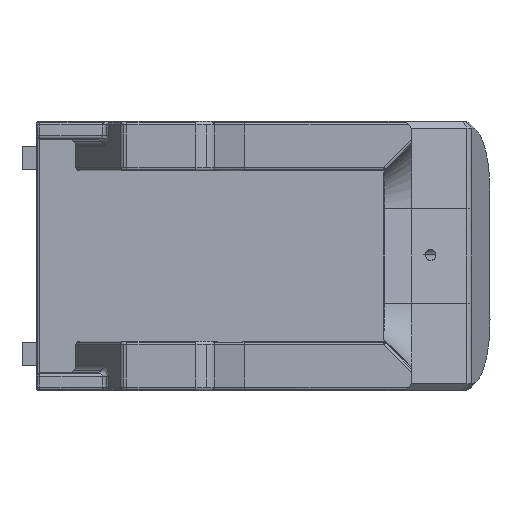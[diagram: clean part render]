
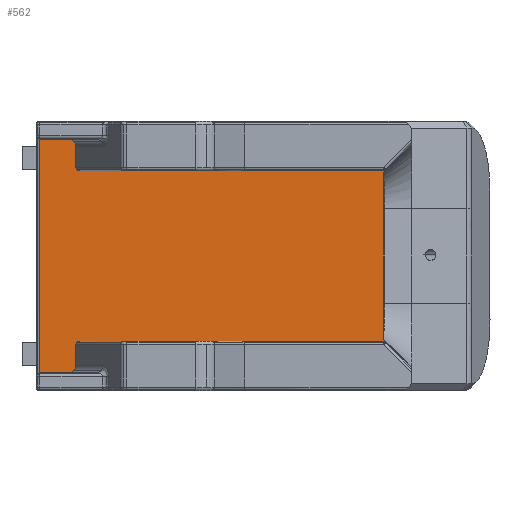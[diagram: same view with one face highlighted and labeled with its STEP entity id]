
A CAD part, left-side view. The second image highlights one B-rep face of the part: STEP entity #562.
In plain terms, the highlighted planar face has unit normal (-1, 0, 0).
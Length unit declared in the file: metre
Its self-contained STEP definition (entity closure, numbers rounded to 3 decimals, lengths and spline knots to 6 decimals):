
#562=ADVANCED_FACE('0:72',(#1731),#1732,.F.);
#1731=FACE_OUTER_BOUND('',#7564,.T.);
#1732=PLANE('',#7565);
#7564=EDGE_LOOP('',(#12483,#12484,#12485,#12486,#12487,#12488,#12489,#12490,#12491,#12492,#12493,#12494,#12495,#12496,#12497,#12498,#12499,#12500,#12501,#12502,#12503,#12504));
#7565=AXIS2_PLACEMENT_3D('',#12505,#12506,#12507);
#12483=ORIENTED_EDGE('',*,*,#14951,.F.);
#12484=ORIENTED_EDGE('',*,*,#13797,.F.);
#12485=ORIENTED_EDGE('',*,*,#14913,.F.);
#12486=ORIENTED_EDGE('',*,*,#14964,.T.);
#12487=ORIENTED_EDGE('',*,*,#14910,.T.);
#12488=ORIENTED_EDGE('',*,*,#13803,.T.);
#12489=ORIENTED_EDGE('',*,*,#15021,.F.);
#12490=ORIENTED_EDGE('',*,*,#15022,.F.);
#12491=ORIENTED_EDGE('',*,*,#15023,.F.);
#12492=ORIENTED_EDGE('',*,*,#13785,.T.);
#12493=ORIENTED_EDGE('',*,*,#14929,.T.);
#12494=ORIENTED_EDGE('',*,*,#15024,.T.);
#12495=ORIENTED_EDGE('',*,*,#14930,.F.);
#12496=ORIENTED_EDGE('',*,*,#13783,.F.);
#12497=ORIENTED_EDGE('',*,*,#15025,.F.);
#12498=ORIENTED_EDGE('',*,*,#13758,.F.);
#12499=ORIENTED_EDGE('',*,*,#14950,.F.);
#12500=ORIENTED_EDGE('',*,*,#15026,.F.);
#12501=ORIENTED_EDGE('',*,*,#14947,.T.);
#12502=ORIENTED_EDGE('',*,*,#14957,.F.);
#12503=ORIENTED_EDGE('',*,*,#13805,.F.);
#12504=ORIENTED_EDGE('',*,*,#14909,.F.);
#12505=CARTESIAN_POINT('',(-0.16753,-0.031141,0.001));
#12506=DIRECTION('',(1.0,0.,0.));
#12507=DIRECTION('',(0.,1.0,0.0));
#13758=EDGE_CURVE('0:1620',#15643,#15646,#15647,.T.);
#13783=EDGE_CURVE('0:1833',#15688,#15684,#15690,.T.);
#13785=EDGE_CURVE('0:1827',#15694,#15691,#15695,.T.);
#13797=EDGE_CURVE('0:1809',#15714,#15717,#15718,.T.);
#13803=EDGE_CURVE('0:1815',#15723,#15727,#15729,.T.);
#13805=EDGE_CURVE('0:1722',#15730,#15733,#15734,.T.);
#14909=EDGE_CURVE('0:1722',#17521,#15730,#17523,.T.);
#14910=EDGE_CURVE('0:1815',#17524,#15723,#17525,.T.);
#14913=EDGE_CURVE('0:1809',#17527,#15714,#17529,.T.);
#14929=EDGE_CURVE('0:1827',#15691,#17549,#17551,.T.);
#14930=EDGE_CURVE('0:1833',#15684,#17552,#17553,.T.);
#14947=EDGE_CURVE('0:1839',#17577,#17575,#17578,.T.);
#14950=EDGE_CURVE('0:1620',#17580,#15643,#17582,.T.);
#14951=EDGE_CURVE('0:1758',#15717,#17521,#17583,.T.);
#14957=EDGE_CURVE('0:1842',#15733,#17575,#17590,.T.);
#14964=EDGE_CURVE('0:1812',#17527,#17524,#17598,.T.);
#15021=EDGE_CURVE('0:1818',#15328,#15727,#17685,.T.);
#15022=EDGE_CURVE('0:1821',#17686,#15328,#17687,.T.);
#15023=EDGE_CURVE('0:1824',#15694,#17686,#17688,.T.);
#15024=EDGE_CURVE('0:1830',#17549,#17552,#17689,.T.);
#15025=EDGE_CURVE('0:1836',#15646,#15688,#17690,.T.);
#15026=EDGE_CURVE('0:1641',#17577,#17580,#17691,.T.);
#15328=VERTEX_POINT('NONE',#18089);
#15643=VERTEX_POINT('',#18612);
#15646=VERTEX_POINT('NONE',#18616);
#15647=CIRCLE('',#18617,0.0005);
#15684=VERTEX_POINT('',#18672);
#15688=VERTEX_POINT('NONE',#18677);
#15690=ELLIPSE('',#18680,0.000577,0.0005);
#15691=VERTEX_POINT('',#18681);
#15694=VERTEX_POINT('NONE',#18685);
#15695=ELLIPSE('',#18686,0.001155,0.001);
#15714=VERTEX_POINT('',#18725);
#15717=VERTEX_POINT('NONE',#18729);
#15718=ELLIPSE('',#18730,0.000577,0.0005);
#15723=VERTEX_POINT('',#18736);
#15727=VERTEX_POINT('NONE',#18745);
#15729=ELLIPSE('',#18748,0.001155,0.001);
#15730=VERTEX_POINT('',#18749);
#15733=VERTEX_POINT('NONE',#18753);
#15734=CIRCLE('',#18754,0.0005);
#17521=VERTEX_POINT('NONE',#23033);
#17523=CIRCLE('',#23036,0.0005);
#17524=VERTEX_POINT('NONE',#23037);
#17525=ELLIPSE('',#23038,0.001155,0.001);
#17527=VERTEX_POINT('NONE',#23041);
#17529=ELLIPSE('',#23044,0.000577,0.0005);
#17549=VERTEX_POINT('NONE',#23093);
#17551=ELLIPSE('',#23096,0.001155,0.001);
#17552=VERTEX_POINT('NONE',#23097);
#17553=ELLIPSE('',#23098,0.000577,0.0005);
#17575=VERTEX_POINT('NONE',#23129);
#17577=VERTEX_POINT('NONE',#23132);
#17578=LINE('',#23133,#23134);
#17580=VERTEX_POINT('NONE',#23137);
#17582=CIRCLE('',#23140,0.0005);
#17583=LINE('',#23141,#23142);
#17590=LINE('',#23155,#23156);
#17598=LINE('',#23168,#23169);
#17685=LINE('',#23385,#23386);
#17686=VERTEX_POINT('NONE',#23387);
#17687=LINE('',#23388,#23389);
#17688=LINE('',#23390,#23391);
#17689=LINE('',#23392,#23393);
#17690=LINE('',#23394,#23395);
#17691=LINE('',#23396,#23397);
#18089=CARTESIAN_POINT('',(-0.16753,-0.00879,0.0175));
#18612=CARTESIAN_POINT('',(-0.16753,-0.057524,-0.011038));
#18616=CARTESIAN_POINT('',(-0.16753,-0.057332,-0.011));
#18617=AXIS2_PLACEMENT_3D('',#24233,#24234,#24235);
#18672=CARTESIAN_POINT('',(-0.16753,-0.014076,-0.011146));
#18677=CARTESIAN_POINT('',(-0.16753,-0.014485,-0.011));
#18680=AXIS2_PLACEMENT_3D('',#24280,#24281,#24282);
#18681=CARTESIAN_POINT('',(-0.16753,-0.013569,-0.015207));
#18685=CARTESIAN_POINT('',(-0.16753,-0.012753,-0.0155));
#18686=AXIS2_PLACEMENT_3D('',#24284,#24285,#24286);
#18725=CARTESIAN_POINT('',(-0.16753,-0.014076,0.013146));
#18729=CARTESIAN_POINT('',(-0.16753,-0.014485,0.013));
#18730=AXIS2_PLACEMENT_3D('',#24299,#24300,#24301);
#18736=CARTESIAN_POINT('',(-0.16753,-0.013569,0.017207));
#18745=CARTESIAN_POINT('',(-0.16753,-0.012753,0.0175));
#18748=AXIS2_PLACEMENT_3D('',#24308,#24309,#24310);
#18749=CARTESIAN_POINT('',(-0.16753,-0.057524,0.013038));
#18753=CARTESIAN_POINT('',(-0.16753,-0.057686,0.013146));
#18754=AXIS2_PLACEMENT_3D('',#24312,#24313,#24314);
#23033=CARTESIAN_POINT('',(-0.16753,-0.057333,0.013));
#23036=AXIS2_PLACEMENT_3D('',#26068,#26069,#26070);
#23037=CARTESIAN_POINT('',(-0.16753,-0.013907,0.0165));
#23038=AXIS2_PLACEMENT_3D('',#26071,#26072,#26073);
#23041=CARTESIAN_POINT('',(-0.16753,-0.013907,0.0135));
#23044=AXIS2_PLACEMENT_3D('',#26076,#26077,#26078);
#23093=CARTESIAN_POINT('',(-0.16753,-0.013907,-0.0145));
#23096=AXIS2_PLACEMENT_3D('',#26101,#26102,#26103);
#23097=CARTESIAN_POINT('',(-0.16753,-0.013907,-0.0115));
#23098=AXIS2_PLACEMENT_3D('',#26104,#26105,#26106);
#23129=CARTESIAN_POINT('',(-0.16753,-0.05729,0.01275));
#23132=CARTESIAN_POINT('',(-0.16753,-0.05729,-0.01075));
#23133=CARTESIAN_POINT('',(-0.16753,-0.05729,0.00917));
#23134=VECTOR('',#26142,1.0);
#23137=CARTESIAN_POINT('',(-0.16753,-0.057686,-0.011146));
#23140=AXIS2_PLACEMENT_3D('',#26145,#26146,#26147);
#23141=CARTESIAN_POINT('',(-0.16753,-0.03284,0.013));
#23142=VECTOR('',#26148,1.0);
#23155=CARTESIAN_POINT('',(-0.16753,-0.048815,0.004275));
#23156=VECTOR('',#26155,1.0);
#23168=CARTESIAN_POINT('',(-0.16753,-0.013907,-0.0091));
#23169=VECTOR('',#26166,1.0);
#23385=CARTESIAN_POINT('',(-0.16753,-0.03284,0.0175));
#23386=VECTOR('',#26224,1.0);
#23387=CARTESIAN_POINT('',(-0.16753,-0.008788,-0.0155));
#23388=CARTESIAN_POINT('',(-0.16753,-0.00879,0.001));
#23389=VECTOR('',#26225,1.0);
#23390=CARTESIAN_POINT('',(-0.16753,-0.031547,-0.0155));
#23391=VECTOR('',#26226,1.0);
#23392=CARTESIAN_POINT('',(-0.16753,-0.013907,-0.0091));
#23393=VECTOR('',#26227,1.0);
#23394=CARTESIAN_POINT('',(-0.16753,-0.031547,-0.011));
#23395=VECTOR('',#26228,1.0);
#23396=CARTESIAN_POINT('',(-0.16753,-0.048815,-0.002275));
#23397=VECTOR('',#26229,1.0);
#24233=CARTESIAN_POINT('',(-0.16753,-0.057332,-0.0115));
#24234=DIRECTION('',(-1.0,0.,0.));
#24235=DIRECTION('',(0.0,-0.383,0.924));
#24280=CARTESIAN_POINT('',(-0.16753,-0.014485,-0.0115));
#24281=DIRECTION('',(-1.0,0.,0.));
#24282=DIRECTION('',(0.,1.0,0.));
#24284=CARTESIAN_POINT('',(-0.16753,-0.012753,-0.0145));
#24285=DIRECTION('',(-1.0,0.0,0.));
#24286=DIRECTION('',(0.,1.0,0.));
#24299=CARTESIAN_POINT('',(-0.16753,-0.014485,0.0135));
#24300=DIRECTION('',(-1.0,0.0,0.));
#24301=DIRECTION('',(0.,1.0,0.));
#24308=CARTESIAN_POINT('',(-0.16753,-0.012753,0.0165));
#24309=DIRECTION('',(-1.0,0.0,0.));
#24310=DIRECTION('',(0.,1.0,0.));
#24312=CARTESIAN_POINT('',(-0.16753,-0.057333,0.0135));
#24313=DIRECTION('',(-1.0,0.,0.));
#24314=DIRECTION('',(0.0,-0.383,-0.924));
#26068=CARTESIAN_POINT('',(-0.16753,-0.057333,0.0135));
#26069=DIRECTION('',(-1.0,0.,0.));
#26070=DIRECTION('',(0.0,-0.383,-0.924));
#26071=CARTESIAN_POINT('',(-0.16753,-0.012753,0.0165));
#26072=DIRECTION('',(-1.0,0.0,0.));
#26073=DIRECTION('',(0.,1.0,0.));
#26076=CARTESIAN_POINT('',(-0.16753,-0.014485,0.0135));
#26077=DIRECTION('',(-1.0,0.0,0.));
#26078=DIRECTION('',(0.,1.0,0.));
#26101=CARTESIAN_POINT('',(-0.16753,-0.012753,-0.0145));
#26102=DIRECTION('',(-1.0,0.0,0.));
#26103=DIRECTION('',(0.,1.0,0.));
#26104=CARTESIAN_POINT('',(-0.16753,-0.014485,-0.0115));
#26105=DIRECTION('',(-1.0,0.,0.));
#26106=DIRECTION('',(0.,1.0,0.));
#26142=DIRECTION('',(0.,0.,1.0));
#26145=CARTESIAN_POINT('',(-0.16753,-0.057332,-0.0115));
#26146=DIRECTION('',(-1.0,0.,0.));
#26147=DIRECTION('',(0.0,-0.383,0.924));
#26148=DIRECTION('',(0.,-1.0,0.));
#26155=DIRECTION('',(0.,0.707,-0.707));
#26166=DIRECTION('',(0.,0.,1.0));
#26224=DIRECTION('',(0.,-1.0,0.));
#26225=DIRECTION('',(0.,0.,1.0));
#26226=DIRECTION('',(0.,1.0,0.));
#26227=DIRECTION('',(0.,0.,1.0));
#26228=DIRECTION('',(0.,1.0,0.));
#26229=DIRECTION('',(0.,-0.707,-0.707));
